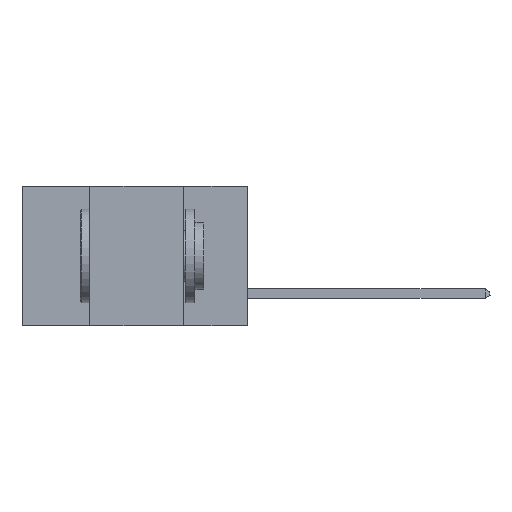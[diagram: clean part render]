
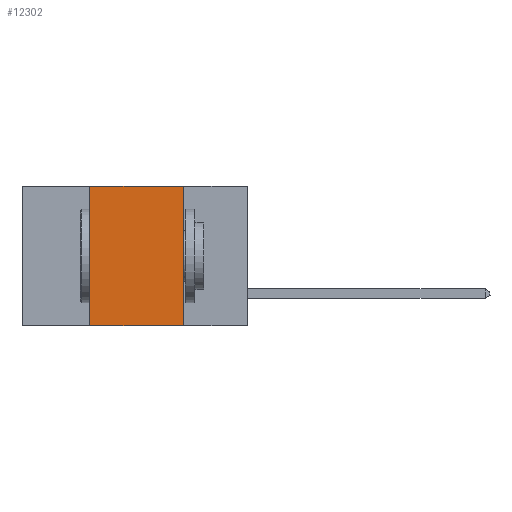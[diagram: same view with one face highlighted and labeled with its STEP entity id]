
A CAD part, left-side view. The second image highlights one B-rep face of the part: STEP entity #12302.
In plain terms, the highlighted planar face has unit normal (-1, 0, 0).
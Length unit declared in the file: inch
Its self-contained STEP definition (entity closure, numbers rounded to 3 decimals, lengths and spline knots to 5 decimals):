
#209 = EDGE_CURVE ( 'NONE', #11658, #5844, #433, .T. ) ;
#433 = LINE ( 'NONE', #3455, #12923 ) ;
#1200 = CARTESIAN_POINT ( 'NONE',  ( 0., 0.6, 0. ) ) ;
#1273 = CARTESIAN_POINT ( 'NONE',  ( 0., 0.42, 0. ) ) ;
#1590 = DIRECTION ( 'NONE',  ( 0., 0., -1. ) ) ;
#1959 = EDGE_LOOP ( 'NONE', ( #4035, #14223, #6651, #10436 ) ) ;
#3455 = CARTESIAN_POINT ( 'NONE',  ( 0., 0.17, 0. ) ) ;
#4035 = ORIENTED_EDGE ( 'NONE', *, *, #209, .F. ) ;
#4390 = EDGE_CURVE ( 'NONE', #14151, #5844, #8946, .T. ) ;
#4446 = PLANE ( 'NONE',  #13993 ) ;
#5533 = VECTOR ( 'NONE', #13674, 39.37008 ) ;
#5723 = LINE ( 'NONE', #8761, #5533 ) ;
#5841 = DIRECTION ( 'NONE',  ( 0., 0., -1. ) ) ;
#5844 = VERTEX_POINT ( 'NONE', #13450 ) ;
#5871 = CARTESIAN_POINT ( 'NONE',  ( 0., 0.6, -0.37 ) ) ;
#6391 = FACE_OUTER_BOUND ( 'NONE', #1959, .T. ) ;
#6651 = ORIENTED_EDGE ( 'NONE', *, *, #9926, .F. ) ;
#7158 = DIRECTION ( 'NONE',  ( 1., 0., 0. ) ) ;
#7291 = VECTOR ( 'NONE', #9084, 39.37008 ) ;
#8009 = CARTESIAN_POINT ( 'NONE',  ( 0., 0.6, 0. ) ) ;
#8761 = CARTESIAN_POINT ( 'NONE',  ( 0., 0.42, 0. ) ) ;
#8946 = LINE ( 'NONE', #5871, #15265 ) ;
#9084 = DIRECTION ( 'NONE',  ( 0., -1., 0. ) ) ;
#9654 = DIRECTION ( 'NONE',  ( 0., -1., 0. ) ) ;
#9926 = EDGE_CURVE ( 'NONE', #14151, #12527, #5723, .T. ) ;
#10435 = LINE ( 'NONE', #8009, #7291 ) ;
#10436 = ORIENTED_EDGE ( 'NONE', *, *, #4390, .T. ) ;
#10835 = CARTESIAN_POINT ( 'NONE',  ( 0., 0.42, -0.37 ) ) ;
#11638 = CARTESIAN_POINT ( 'NONE',  ( 0., 0.17, 0. ) ) ;
#11658 = VERTEX_POINT ( 'NONE', #11638 ) ;
#12302 = ADVANCED_FACE ( 'NONE', ( #6391 ), #4446, .F. ) ;
#12527 = VERTEX_POINT ( 'NONE', #1273 ) ;
#12923 = VECTOR ( 'NONE', #5841, 39.37008 ) ;
#13450 = CARTESIAN_POINT ( 'NONE',  ( 0., 0.17, -0.37 ) ) ;
#13674 = DIRECTION ( 'NONE',  ( 0., 0., 1. ) ) ;
#13912 = EDGE_CURVE ( 'NONE', #12527, #11658, #10435, .T. ) ;
#13993 = AXIS2_PLACEMENT_3D ( 'NONE', #1200, #7158, #1590 ) ;
#14151 = VERTEX_POINT ( 'NONE', #10835 ) ;
#14223 = ORIENTED_EDGE ( 'NONE', *, *, #13912, .F. ) ;
#15265 = VECTOR ( 'NONE', #9654, 39.37008 ) ;
